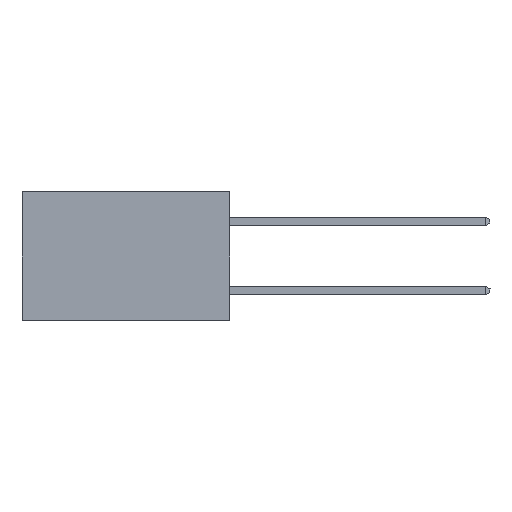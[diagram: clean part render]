
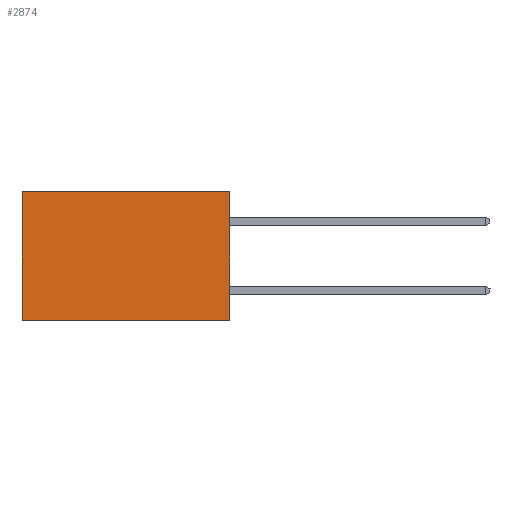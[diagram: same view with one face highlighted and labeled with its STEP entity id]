
A CAD part, left-side view. The second image highlights one B-rep face of the part: STEP entity #2874.
In plain terms, the highlighted planar face has unit normal (-1, 0, 0).
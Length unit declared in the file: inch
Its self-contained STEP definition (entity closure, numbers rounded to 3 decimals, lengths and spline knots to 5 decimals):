
#30 = EDGE_CURVE ( 'NONE', #15372, #22911, #21722, .T. ) ;
#1163 = VECTOR ( 'NONE', #1361, 39.37008 ) ;
#1361 = DIRECTION ( 'NONE',  ( 0., 1., 0. ) ) ;
#2196 = ORIENTED_EDGE ( 'NONE', *, *, #12530, .F. ) ;
#2874 = ADVANCED_FACE ( 'NONE', ( #23055 ), #5979, .F. ) ;
#3905 = VERTEX_POINT ( 'NONE', #5559 ) ;
#4566 = CARTESIAN_POINT ( 'NONE',  ( 0.2615, 0.6, -0.37 ) ) ;
#4842 = VECTOR ( 'NONE', #24330, 39.37008 ) ;
#5409 = DIRECTION ( 'NONE',  ( 0., 0., -1. ) ) ;
#5421 = LINE ( 'NONE', #22179, #27093 ) ;
#5559 = CARTESIAN_POINT ( 'NONE',  ( 0.2615, 0., -0.37 ) ) ;
#5599 = DIRECTION ( 'NONE',  ( 1., 0., 0. ) ) ;
#5948 = CARTESIAN_POINT ( 'NONE',  ( 0.2615, 0., -0.37 ) ) ;
#5978 = EDGE_LOOP ( 'NONE', ( #19518, #21814, #2196, #17691 ) ) ;
#5979 = PLANE ( 'NONE',  #7874 ) ;
#6237 = LINE ( 'NONE', #14189, #1163 ) ;
#7874 = AXIS2_PLACEMENT_3D ( 'NONE', #5948, #5599, #5409 ) ;
#8878 = VERTEX_POINT ( 'NONE', #9017 ) ;
#9017 = CARTESIAN_POINT ( 'NONE',  ( 0.2615, 0.6, -0.37 ) ) ;
#9758 = CARTESIAN_POINT ( 'NONE',  ( 0.2615, 0., 0. ) ) ;
#11092 = LINE ( 'NONE', #4566, #27081 ) ;
#12530 = EDGE_CURVE ( 'NONE', #15372, #3905, #5421, .T. ) ;
#13668 = CARTESIAN_POINT ( 'NONE',  ( 0.2615, 0.6, 0. ) ) ;
#13856 = DIRECTION ( 'NONE',  ( 0., 0., -1. ) ) ;
#14189 = CARTESIAN_POINT ( 'NONE',  ( 0.2615, 0., -0.37 ) ) ;
#15372 = VERTEX_POINT ( 'NONE', #26133 ) ;
#17691 = ORIENTED_EDGE ( 'NONE', *, *, #30, .T. ) ;
#19518 = ORIENTED_EDGE ( 'NONE', *, *, #25748, .T. ) ;
#21722 = LINE ( 'NONE', #9758, #4842 ) ;
#21814 = ORIENTED_EDGE ( 'NONE', *, *, #23736, .F. ) ;
#22179 = CARTESIAN_POINT ( 'NONE',  ( 0.2615, 0., -0.37 ) ) ;
#22911 = VERTEX_POINT ( 'NONE', #13668 ) ;
#23055 = FACE_OUTER_BOUND ( 'NONE', #5978, .T. ) ;
#23736 = EDGE_CURVE ( 'NONE', #3905, #8878, #6237, .T. ) ;
#24330 = DIRECTION ( 'NONE',  ( 0., 1., 0. ) ) ;
#25628 = DIRECTION ( 'NONE',  ( 0., 0., -1. ) ) ;
#25748 = EDGE_CURVE ( 'NONE', #22911, #8878, #11092, .T. ) ;
#26133 = CARTESIAN_POINT ( 'NONE',  ( 0.2615, 0., 0. ) ) ;
#27081 = VECTOR ( 'NONE', #25628, 39.37008 ) ;
#27093 = VECTOR ( 'NONE', #13856, 39.37008 ) ;
